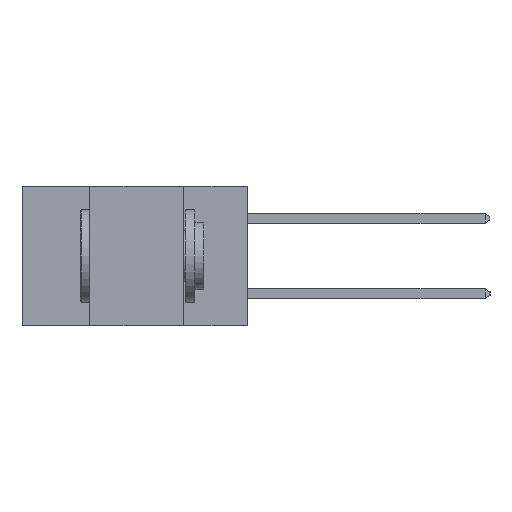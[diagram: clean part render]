
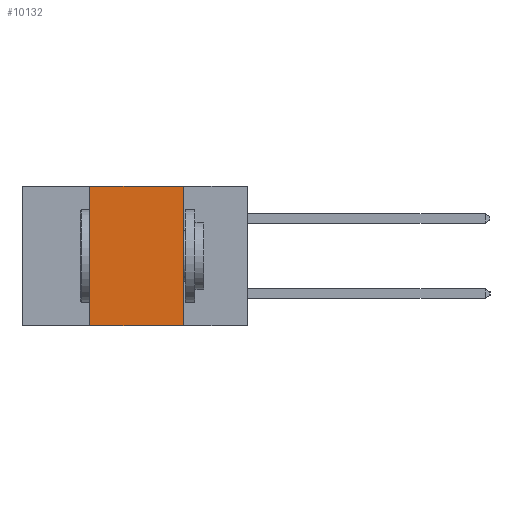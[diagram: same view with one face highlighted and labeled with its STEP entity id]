
A CAD part, left-side view. The second image highlights one B-rep face of the part: STEP entity #10132.
In plain terms, the highlighted planar face has unit normal (-1, 0, 0).
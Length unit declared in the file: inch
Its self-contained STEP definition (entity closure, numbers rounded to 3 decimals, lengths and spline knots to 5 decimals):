
#471 = EDGE_CURVE ( 'NONE', #16551, #22196, #2674, .T. ) ;
#1519 = CARTESIAN_POINT ( 'NONE',  ( 0., 0.42, 0. ) ) ;
#2243 = PLANE ( 'NONE',  #14949 ) ;
#2674 = LINE ( 'NONE', #17229, #23244 ) ;
#3319 = CARTESIAN_POINT ( 'NONE',  ( 0., 0.17, 0. ) ) ;
#4537 = LINE ( 'NONE', #21824, #15183 ) ;
#6736 = CARTESIAN_POINT ( 'NONE',  ( 0., 0.17, -0.37 ) ) ;
#6861 = VERTEX_POINT ( 'NONE', #1519 ) ;
#7359 = EDGE_CURVE ( 'NONE', #16551, #6861, #4537, .T. ) ;
#8400 = DIRECTION ( 'NONE',  ( 1., 0., 0. ) ) ;
#8540 = ORIENTED_EDGE ( 'NONE', *, *, #7359, .F. ) ;
#9157 = FACE_OUTER_BOUND ( 'NONE', #21997, .T. ) ;
#9370 = ORIENTED_EDGE ( 'NONE', *, *, #17928, .F. ) ;
#9441 = ORIENTED_EDGE ( 'NONE', *, *, #471, .T. ) ;
#10132 = ADVANCED_FACE ( 'NONE', ( #9157 ), #2243, .F. ) ;
#12216 = CARTESIAN_POINT ( 'NONE',  ( 0., 0.17, -0.37 ) ) ;
#13181 = CARTESIAN_POINT ( 'NONE',  ( 0., 0.6, 0. ) ) ;
#13326 = VECTOR ( 'NONE', #25008, 39.37008 ) ;
#13913 = LINE ( 'NONE', #13181, #13326 ) ;
#14287 = CARTESIAN_POINT ( 'NONE',  ( 0., 0.6, 0. ) ) ;
#14949 = AXIS2_PLACEMENT_3D ( 'NONE', #14287, #8400, #22223 ) ;
#15002 = CARTESIAN_POINT ( 'NONE',  ( 0., 0.42, -0.37 ) ) ;
#15183 = VECTOR ( 'NONE', #24340, 39.37008 ) ;
#15336 = EDGE_CURVE ( 'NONE', #6861, #20476, #13913, .T. ) ;
#16551 = VERTEX_POINT ( 'NONE', #15002 ) ;
#17089 = DIRECTION ( 'NONE',  ( 0., -1., 0. ) ) ;
#17229 = CARTESIAN_POINT ( 'NONE',  ( 0., 0.6, -0.37 ) ) ;
#17928 = EDGE_CURVE ( 'NONE', #20476, #22196, #18012, .T. ) ;
#18012 = LINE ( 'NONE', #12216, #19222 ) ;
#18492 = ORIENTED_EDGE ( 'NONE', *, *, #15336, .F. ) ;
#19222 = VECTOR ( 'NONE', #19973, 39.37008 ) ;
#19973 = DIRECTION ( 'NONE',  ( 0., 0., -1. ) ) ;
#20476 = VERTEX_POINT ( 'NONE', #3319 ) ;
#21824 = CARTESIAN_POINT ( 'NONE',  ( 0., 0.42, -0.37 ) ) ;
#21997 = EDGE_LOOP ( 'NONE', ( #9370, #18492, #8540, #9441 ) ) ;
#22196 = VERTEX_POINT ( 'NONE', #6736 ) ;
#22223 = DIRECTION ( 'NONE',  ( 0., 0., -1. ) ) ;
#23244 = VECTOR ( 'NONE', #17089, 39.37008 ) ;
#24340 = DIRECTION ( 'NONE',  ( 0., 0., 1. ) ) ;
#25008 = DIRECTION ( 'NONE',  ( 0., -1., 0. ) ) ;
